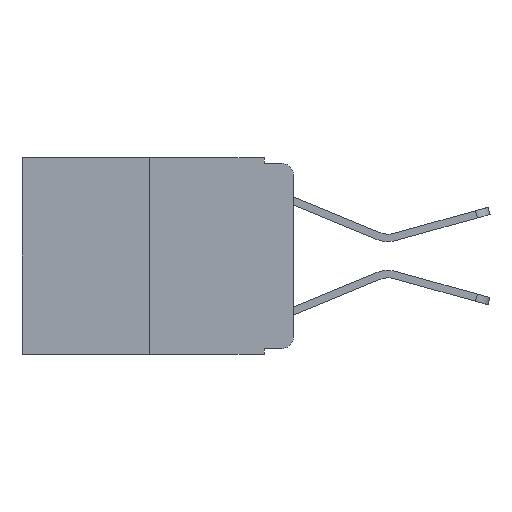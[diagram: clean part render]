
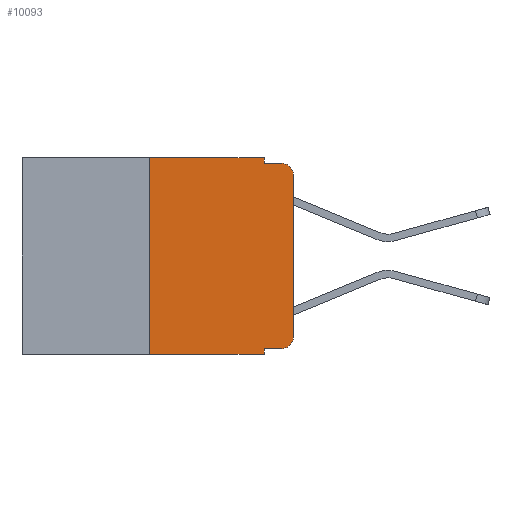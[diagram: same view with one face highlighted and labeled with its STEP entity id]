
A CAD part, left-side view. The second image highlights one B-rep face of the part: STEP entity #10093.
In plain terms, the highlighted planar face has unit normal (-1, 0, 0).
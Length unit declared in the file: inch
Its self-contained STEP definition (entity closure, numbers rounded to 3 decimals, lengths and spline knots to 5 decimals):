
#19 = VERTEX_POINT ( 'NONE', #13531 ) ;
#108 = DIRECTION ( 'NONE',  ( -1., 0., 0. ) ) ;
#244 = DIRECTION ( 'NONE',  ( 0., 0., -1. ) ) ;
#541 = ORIENTED_EDGE ( 'NONE', *, *, #3503, .F. ) ;
#580 = AXIS2_PLACEMENT_3D ( 'NONE', #10492, #108, #9292 ) ;
#602 = ORIENTED_EDGE ( 'NONE', *, *, #9617, .F. ) ;
#784 = VERTEX_POINT ( 'NONE', #14713 ) ;
#929 = CARTESIAN_POINT ( 'NONE',  ( 0., 0.051, -0.343 ) ) ;
#1093 = VECTOR ( 'NONE', #13517, 39.37008 ) ;
#1522 = EDGE_CURVE ( 'NONE', #2126, #3689, #7058, .T. ) ;
#1700 = EDGE_CURVE ( 'NONE', #19, #11045, #5315, .T. ) ;
#2037 = LINE ( 'NONE', #12428, #2792 ) ;
#2126 = VERTEX_POINT ( 'NONE', #12142 ) ;
#2178 = ORIENTED_EDGE ( 'NONE', *, *, #2864, .T. ) ;
#2308 = LINE ( 'NONE', #10212, #3842 ) ;
#2621 = DIRECTION ( 'NONE',  ( 0., -1., 0. ) ) ;
#2686 = CARTESIAN_POINT ( 'NONE',  ( 0., 0.051, -0.333 ) ) ;
#2716 = AXIS2_PLACEMENT_3D ( 'NONE', #4773, #4998, #244 ) ;
#2792 = VECTOR ( 'NONE', #3474, 39.37008 ) ;
#2844 = DIRECTION ( 'NONE',  ( -1., 0., 0. ) ) ;
#2864 = EDGE_CURVE ( 'NONE', #3689, #784, #8170, .T. ) ;
#2996 = CARTESIAN_POINT ( 'NONE',  ( 0., 0.02, -0.01 ) ) ;
#3019 = ORIENTED_EDGE ( 'NONE', *, *, #5741, .T. ) ;
#3047 = CARTESIAN_POINT ( 'NONE',  ( 0., 0.051, 0. ) ) ;
#3474 = DIRECTION ( 'NONE',  ( 0., 0., 1. ) ) ;
#3503 = EDGE_CURVE ( 'NONE', #2126, #14419, #9666, .T. ) ;
#3689 = VERTEX_POINT ( 'NONE', #4694 ) ;
#3842 = VECTOR ( 'NONE', #4340, 39.37008 ) ;
#4318 = EDGE_CURVE ( 'NONE', #9553, #19, #2308, .T. ) ;
#4340 = DIRECTION ( 'NONE',  ( 0., 0., -1. ) ) ;
#4694 = CARTESIAN_POINT ( 'NONE',  ( 0., 0.02, -0.333 ) ) ;
#4773 = CARTESIAN_POINT ( 'NONE',  ( 0., 0.473, 0. ) ) ;
#4881 = EDGE_CURVE ( 'NONE', #12506, #11045, #6819, .T. ) ;
#4945 = DIRECTION ( 'NONE',  ( 0., -1., 0. ) ) ;
#4998 = DIRECTION ( 'NONE',  ( 1., 0., 0. ) ) ;
#5315 = LINE ( 'NONE', #9901, #11972 ) ;
#5479 = CARTESIAN_POINT ( 'NONE',  ( 0., 0., -0.03 ) ) ;
#5741 = EDGE_CURVE ( 'NONE', #784, #12506, #5950, .T. ) ;
#5834 = LINE ( 'NONE', #6818, #1093 ) ;
#5950 = LINE ( 'NONE', #13788, #11541 ) ;
#6535 = CARTESIAN_POINT ( 'NONE',  ( 0., 0.25, 0. ) ) ;
#6696 = VECTOR ( 'NONE', #4945, 39.37008 ) ;
#6818 = CARTESIAN_POINT ( 'NONE',  ( 0., 0.473, -0.343 ) ) ;
#6819 = CIRCLE ( 'NONE', #580, 0.02 ) ;
#6990 = AXIS2_PLACEMENT_3D ( 'NONE', #14311, #2844, #7359 ) ;
#7058 = LINE ( 'NONE', #2686, #6696 ) ;
#7163 = CARTESIAN_POINT ( 'NONE',  ( 0., 0.051, 0. ) ) ;
#7359 = DIRECTION ( 'NONE',  ( 0., 0., -1. ) ) ;
#7632 = DIRECTION ( 'NONE',  ( 0., 0., -1. ) ) ;
#7846 = VERTEX_POINT ( 'NONE', #12092 ) ;
#8170 = CIRCLE ( 'NONE', #6990, 0.02 ) ;
#8179 = ORIENTED_EDGE ( 'NONE', *, *, #1522, .T. ) ;
#8230 = VECTOR ( 'NONE', #2621, 39.37008 ) ;
#8854 = ORIENTED_EDGE ( 'NONE', *, *, #14401, .T. ) ;
#8928 = ORIENTED_EDGE ( 'NONE', *, *, #14844, .F. ) ;
#9038 = DIRECTION ( 'NONE',  ( 0., 0., 1. ) ) ;
#9292 = DIRECTION ( 'NONE',  ( 0., 0., -1. ) ) ;
#9319 = LINE ( 'NONE', #14078, #8230 ) ;
#9553 = VERTEX_POINT ( 'NONE', #7163 ) ;
#9617 = EDGE_CURVE ( 'NONE', #12365, #9553, #9319, .T. ) ;
#9666 = LINE ( 'NONE', #3047, #9727 ) ;
#9727 = VECTOR ( 'NONE', #7632, 39.37008 ) ;
#9901 = CARTESIAN_POINT ( 'NONE',  ( 0., 0.051, -0.01 ) ) ;
#10093 = ADVANCED_FACE ( 'NONE', ( #12827 ), #11902, .F. ) ;
#10212 = CARTESIAN_POINT ( 'NONE',  ( 0., 0.051, 0. ) ) ;
#10492 = CARTESIAN_POINT ( 'NONE',  ( 0., 0.02, -0.03 ) ) ;
#11045 = VERTEX_POINT ( 'NONE', #2996 ) ;
#11541 = VECTOR ( 'NONE', #9038, 39.37008 ) ;
#11740 = ORIENTED_EDGE ( 'NONE', *, *, #4318, .F. ) ;
#11902 = PLANE ( 'NONE',  #2716 ) ;
#11972 = VECTOR ( 'NONE', #14308, 39.37008 ) ;
#12092 = CARTESIAN_POINT ( 'NONE',  ( 0., 0.25, -0.343 ) ) ;
#12142 = CARTESIAN_POINT ( 'NONE',  ( 0., 0.051, -0.333 ) ) ;
#12365 = VERTEX_POINT ( 'NONE', #6535 ) ;
#12428 = CARTESIAN_POINT ( 'NONE',  ( 0., 0.25, 0. ) ) ;
#12506 = VERTEX_POINT ( 'NONE', #5479 ) ;
#12827 = FACE_OUTER_BOUND ( 'NONE', #12929, .T. ) ;
#12929 = EDGE_LOOP ( 'NONE', ( #3019, #13042, #14334, #11740, #602, #8928, #8854, #541, #8179, #2178 ) ) ;
#13042 = ORIENTED_EDGE ( 'NONE', *, *, #4881, .T. ) ;
#13517 = DIRECTION ( 'NONE',  ( 0., -1., 0. ) ) ;
#13531 = CARTESIAN_POINT ( 'NONE',  ( 0., 0.051, -0.01 ) ) ;
#13788 = CARTESIAN_POINT ( 'NONE',  ( 0., 0., 0. ) ) ;
#14078 = CARTESIAN_POINT ( 'NONE',  ( 0., 0.473, 0. ) ) ;
#14308 = DIRECTION ( 'NONE',  ( 0., -1., 0. ) ) ;
#14311 = CARTESIAN_POINT ( 'NONE',  ( 0., 0.02, -0.313 ) ) ;
#14334 = ORIENTED_EDGE ( 'NONE', *, *, #1700, .F. ) ;
#14401 = EDGE_CURVE ( 'NONE', #7846, #14419, #5834, .T. ) ;
#14419 = VERTEX_POINT ( 'NONE', #929 ) ;
#14713 = CARTESIAN_POINT ( 'NONE',  ( 0., 0., -0.313 ) ) ;
#14844 = EDGE_CURVE ( 'NONE', #7846, #12365, #2037, .T. ) ;
